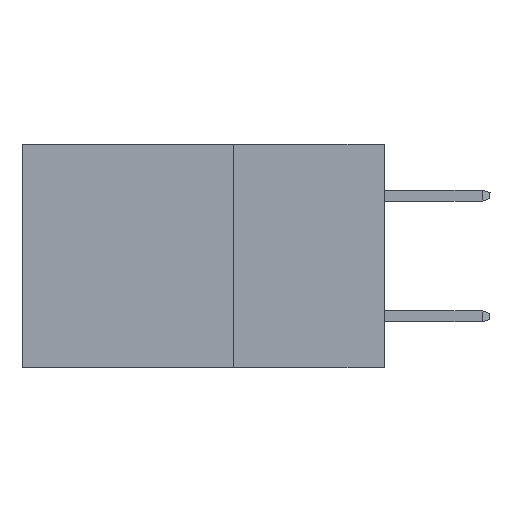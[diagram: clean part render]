
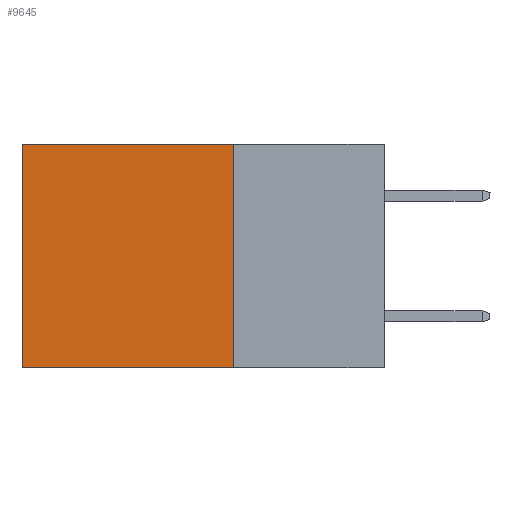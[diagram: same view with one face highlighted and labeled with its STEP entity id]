
A CAD part, left-side view. The second image highlights one B-rep face of the part: STEP entity #9645.
In plain terms, the highlighted planar face has unit normal (-1, 0, 0).
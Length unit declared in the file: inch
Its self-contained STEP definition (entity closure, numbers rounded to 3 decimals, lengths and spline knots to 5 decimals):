
#1551 = DIRECTION ( 'NONE',  ( 0., 0., -1. ) ) ;
#2712 = ORIENTED_EDGE ( 'NONE', *, *, #13174, .T. ) ;
#3359 = DIRECTION ( 'NONE',  ( 0., 1., 0. ) ) ;
#3546 = CARTESIAN_POINT ( 'NONE',  ( 0.298, 0.25, 0. ) ) ;
#4655 = CARTESIAN_POINT ( 'NONE',  ( 0.298, 0.6, -0.37 ) ) ;
#5781 = CARTESIAN_POINT ( 'NONE',  ( 0.298, 0.25, 0. ) ) ;
#6140 = PLANE ( 'NONE',  #18979 ) ;
#8786 = LINE ( 'NONE', #3546, #10843 ) ;
#8831 = VERTEX_POINT ( 'NONE', #20208 ) ;
#9645 = ADVANCED_FACE ( 'NONE', ( #24430 ), #6140, .F. ) ;
#10138 = DIRECTION ( 'NONE',  ( 0., 0., -1. ) ) ;
#10843 = VECTOR ( 'NONE', #14222, 39.37008 ) ;
#10960 = VECTOR ( 'NONE', #3359, 39.37008 ) ;
#10989 = ORIENTED_EDGE ( 'NONE', *, *, #13565, .F. ) ;
#11168 = VERTEX_POINT ( 'NONE', #24886 ) ;
#12332 = LINE ( 'NONE', #25277, #10960 ) ;
#13174 = EDGE_CURVE ( 'NONE', #18098, #11168, #8786, .T. ) ;
#13565 = EDGE_CURVE ( 'NONE', #18098, #8831, #26047, .T. ) ;
#13718 = ORIENTED_EDGE ( 'NONE', *, *, #17845, .T. ) ;
#14064 = CARTESIAN_POINT ( 'NONE',  ( 0.298, 0.6, 0. ) ) ;
#14222 = DIRECTION ( 'NONE',  ( 0., 1., 0. ) ) ;
#14616 = DIRECTION ( 'NONE',  ( 1., 0., 0. ) ) ;
#15008 = VECTOR ( 'NONE', #18782, 39.37008 ) ;
#16446 = EDGE_LOOP ( 'NONE', ( #13718, #23413, #10989, #2712 ) ) ;
#16821 = EDGE_CURVE ( 'NONE', #8831, #18221, #12332, .T. ) ;
#17845 = EDGE_CURVE ( 'NONE', #11168, #18221, #27853, .T. ) ;
#18098 = VERTEX_POINT ( 'NONE', #21668 ) ;
#18221 = VERTEX_POINT ( 'NONE', #4655 ) ;
#18782 = DIRECTION ( 'NONE',  ( 0., 0., -1. ) ) ;
#18979 = AXIS2_PLACEMENT_3D ( 'NONE', #21433, #14616, #10138 ) ;
#20208 = CARTESIAN_POINT ( 'NONE',  ( 0.298, 0.25, -0.37 ) ) ;
#21433 = CARTESIAN_POINT ( 'NONE',  ( 0.298, 0.25, 0. ) ) ;
#21668 = CARTESIAN_POINT ( 'NONE',  ( 0.298, 0.25, 0. ) ) ;
#22672 = VECTOR ( 'NONE', #1551, 39.37008 ) ;
#23413 = ORIENTED_EDGE ( 'NONE', *, *, #16821, .F. ) ;
#24430 = FACE_OUTER_BOUND ( 'NONE', #16446, .T. ) ;
#24886 = CARTESIAN_POINT ( 'NONE',  ( 0.298, 0.6, 0. ) ) ;
#25277 = CARTESIAN_POINT ( 'NONE',  ( 0.298, 0.25, -0.37 ) ) ;
#26047 = LINE ( 'NONE', #5781, #22672 ) ;
#27853 = LINE ( 'NONE', #14064, #15008 ) ;
